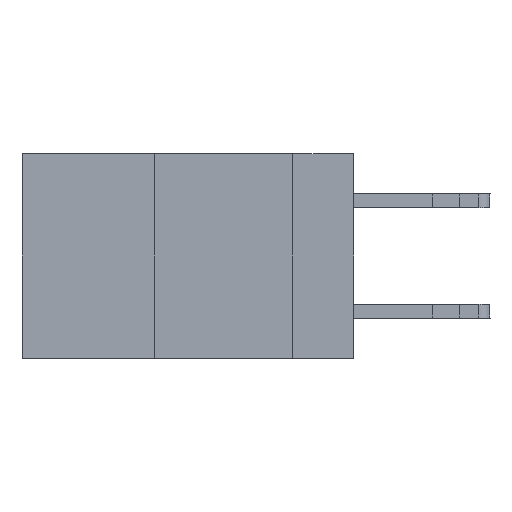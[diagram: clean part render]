
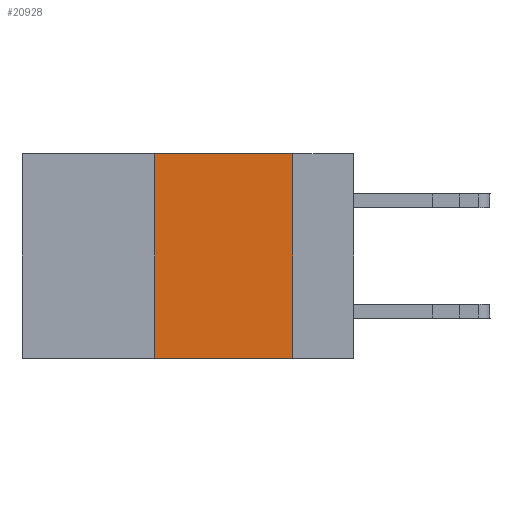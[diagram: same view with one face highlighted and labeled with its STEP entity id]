
A CAD part, left-side view. The second image highlights one B-rep face of the part: STEP entity #20928.
In plain terms, the highlighted planar face has unit normal (-1, 0, 0).
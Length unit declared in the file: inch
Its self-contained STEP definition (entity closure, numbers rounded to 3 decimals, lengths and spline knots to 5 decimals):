
#353 = CARTESIAN_POINT ( 'NONE',  ( 0., 0.36, 0. ) ) ;
#665 = ORIENTED_EDGE ( 'NONE', *, *, #23983, .T. ) ;
#676 = EDGE_LOOP ( 'NONE', ( #21363, #24739, #25833, #665 ) ) ;
#1134 = CARTESIAN_POINT ( 'NONE',  ( 0., 0.6, -0.37 ) ) ;
#1612 = VERTEX_POINT ( 'NONE', #10050 ) ;
#2162 = DIRECTION ( 'NONE',  ( 0., -1., 0. ) ) ;
#2892 = EDGE_CURVE ( 'NONE', #4574, #13466, #29556, .T. ) ;
#4488 = EDGE_CURVE ( 'NONE', #12179, #4574, #14734, .T. ) ;
#4574 = VERTEX_POINT ( 'NONE', #14992 ) ;
#5041 = LINE ( 'NONE', #1134, #28167 ) ;
#8541 = CARTESIAN_POINT ( 'NONE',  ( 0., 0.6, 0. ) ) ;
#9187 = EDGE_CURVE ( 'NONE', #1612, #12179, #10549, .T. ) ;
#10032 = VECTOR ( 'NONE', #20851, 39.37008 ) ;
#10050 = CARTESIAN_POINT ( 'NONE',  ( 0., 0.36, -0.37 ) ) ;
#10549 = LINE ( 'NONE', #353, #27128 ) ;
#10857 = AXIS2_PLACEMENT_3D ( 'NONE', #8541, #17570, #29615 ) ;
#11879 = CARTESIAN_POINT ( 'NONE',  ( 0., 0.36, 0. ) ) ;
#12179 = VERTEX_POINT ( 'NONE', #11879 ) ;
#13466 = VERTEX_POINT ( 'NONE', #28608 ) ;
#14734 = LINE ( 'NONE', #20892, #27605 ) ;
#14992 = CARTESIAN_POINT ( 'NONE',  ( 0., 0.11, 0. ) ) ;
#15747 = CARTESIAN_POINT ( 'NONE',  ( 0., 0.11, 0. ) ) ;
#17570 = DIRECTION ( 'NONE',  ( 1., 0., 0. ) ) ;
#20851 = DIRECTION ( 'NONE',  ( 0., 0., -1. ) ) ;
#20892 = CARTESIAN_POINT ( 'NONE',  ( 0., 0.6, 0. ) ) ;
#20928 = ADVANCED_FACE ( 'NONE', ( #25475 ), #27339, .F. ) ;
#21363 = ORIENTED_EDGE ( 'NONE', *, *, #2892, .F. ) ;
#23657 = DIRECTION ( 'NONE',  ( 0., 0., 1. ) ) ;
#23983 = EDGE_CURVE ( 'NONE', #1612, #13466, #5041, .T. ) ;
#24548 = DIRECTION ( 'NONE',  ( 0., -1., 0. ) ) ;
#24739 = ORIENTED_EDGE ( 'NONE', *, *, #4488, .F. ) ;
#25475 = FACE_OUTER_BOUND ( 'NONE', #676, .T. ) ;
#25833 = ORIENTED_EDGE ( 'NONE', *, *, #9187, .F. ) ;
#27128 = VECTOR ( 'NONE', #23657, 39.37008 ) ;
#27339 = PLANE ( 'NONE',  #10857 ) ;
#27605 = VECTOR ( 'NONE', #2162, 39.37008 ) ;
#28167 = VECTOR ( 'NONE', #24548, 39.37008 ) ;
#28608 = CARTESIAN_POINT ( 'NONE',  ( 0., 0.11, -0.37 ) ) ;
#29556 = LINE ( 'NONE', #15747, #10032 ) ;
#29615 = DIRECTION ( 'NONE',  ( 0., 0., -1. ) ) ;
